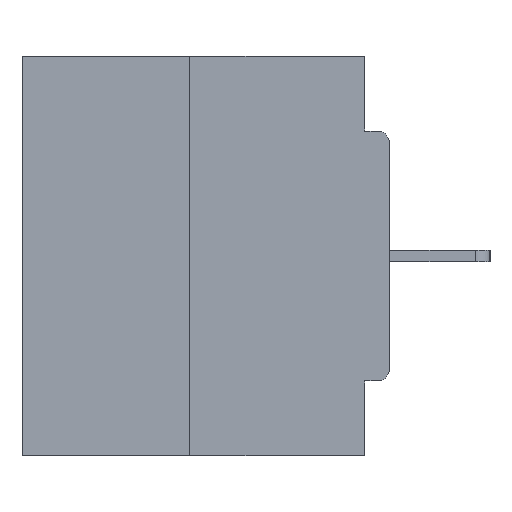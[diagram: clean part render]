
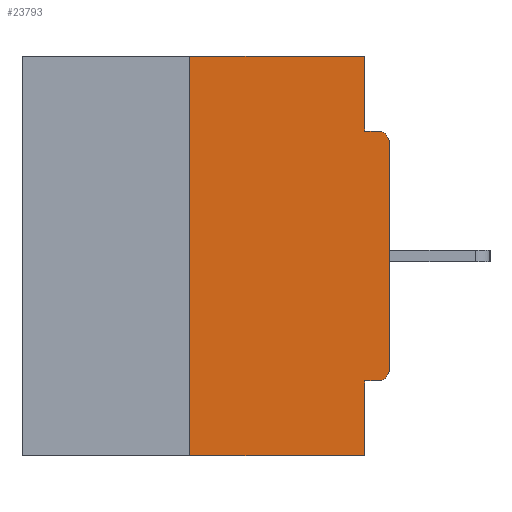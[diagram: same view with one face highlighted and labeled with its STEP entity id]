
A CAD part, left-side view. The second image highlights one B-rep face of the part: STEP entity #23793.
In plain terms, the highlighted planar face has unit normal (-1, 0, 0).
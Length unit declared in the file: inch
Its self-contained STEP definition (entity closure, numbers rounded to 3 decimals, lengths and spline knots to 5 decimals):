
#440 = EDGE_CURVE ( 'NONE', #18291, #3033, #17135, .T. ) ;
#484 = ORIENTED_EDGE ( 'NONE', *, *, #12071, .F. ) ;
#858 = VERTEX_POINT ( 'NONE', #8418 ) ;
#1251 = ORIENTED_EDGE ( 'NONE', *, *, #30407, .F. ) ;
#1846 = CARTESIAN_POINT ( 'NONE',  ( 0., 0.031, -0.5 ) ) ;
#2391 = CARTESIAN_POINT ( 'NONE',  ( 0., 0., -0.1085 ) ) ;
#3033 = VERTEX_POINT ( 'NONE', #1846 ) ;
#3339 = EDGE_CURVE ( 'NONE', #17771, #24456, #18511, .T. ) ;
#3683 = VECTOR ( 'NONE', #10704, 39.37008 ) ;
#3714 = CARTESIAN_POINT ( 'NONE',  ( 0., 0.015, -0.1085 ) ) ;
#4414 = ORIENTED_EDGE ( 'NONE', *, *, #12918, .T. ) ;
#4760 = CARTESIAN_POINT ( 'NONE',  ( 0., 0.46, 0. ) ) ;
#4828 = LINE ( 'NONE', #17891, #10597 ) ;
#4880 = CARTESIAN_POINT ( 'NONE',  ( 0., 0.25, 0. ) ) ;
#5171 = ORIENTED_EDGE ( 'NONE', *, *, #12303, .F. ) ;
#6205 = AXIS2_PLACEMENT_3D ( 'NONE', #26449, #26445, #26379 ) ;
#6224 = DIRECTION ( 'NONE',  ( 0., 0., -1. ) ) ;
#6331 = ORIENTED_EDGE ( 'NONE', *, *, #3339, .F. ) ;
#6459 = VECTOR ( 'NONE', #11971, 39.37008 ) ;
#7105 = ORIENTED_EDGE ( 'NONE', *, *, #440, .T. ) ;
#7230 = DIRECTION ( 'NONE',  ( 1., 0., 0. ) ) ;
#7357 = EDGE_CURVE ( 'NONE', #858, #25612, #29473, .T. ) ;
#7960 = EDGE_LOOP ( 'NONE', ( #6331, #484, #7105, #1251, #27977, #28705, #10176, #4414, #5171, #18187 ) ) ;
#8163 = VERTEX_POINT ( 'NONE', #8510 ) ;
#8179 = DIRECTION ( 'NONE',  ( 0., -1., 0. ) ) ;
#8418 = CARTESIAN_POINT ( 'NONE',  ( 0., 0.015, -0.4065 ) ) ;
#8510 = CARTESIAN_POINT ( 'NONE',  ( 0., 0.031, -0.4065 ) ) ;
#10176 = ORIENTED_EDGE ( 'NONE', *, *, #27878, .T. ) ;
#10597 = VECTOR ( 'NONE', #8179, 39.37008 ) ;
#10667 = VECTOR ( 'NONE', #26387, 39.37008 ) ;
#10704 = DIRECTION ( 'NONE',  ( 0., 1., 0. ) ) ;
#11031 = LINE ( 'NONE', #25330, #3683 ) ;
#11694 = EDGE_CURVE ( 'NONE', #858, #8163, #11031, .T. ) ;
#11783 = LINE ( 'NONE', #4880, #17455 ) ;
#11971 = DIRECTION ( 'NONE',  ( 0., 0., -1. ) ) ;
#12055 = VERTEX_POINT ( 'NONE', #14621 ) ;
#12056 = CARTESIAN_POINT ( 'NONE',  ( 0., 0.46, 0. ) ) ;
#12071 = EDGE_CURVE ( 'NONE', #18291, #17771, #11783, .T. ) ;
#12122 = DIRECTION ( 'NONE',  ( 0., 0., 1. ) ) ;
#12216 = CARTESIAN_POINT ( 'NONE',  ( 0., 0.031, 0. ) ) ;
#12303 = EDGE_CURVE ( 'NONE', #19927, #12055, #4828, .T. ) ;
#12918 = EDGE_CURVE ( 'NONE', #16972, #12055, #25348, .T. ) ;
#14215 = CARTESIAN_POINT ( 'NONE',  ( 0., 0.25, 0. ) ) ;
#14621 = CARTESIAN_POINT ( 'NONE',  ( 0., 0.015, -0.0935 ) ) ;
#15422 = DIRECTION ( 'NONE',  ( 0., -1., 0. ) ) ;
#16074 = CARTESIAN_POINT ( 'NONE',  ( 0., 0.25, -0.5 ) ) ;
#16972 = VERTEX_POINT ( 'NONE', #2391 ) ;
#17135 = LINE ( 'NONE', #25117, #10667 ) ;
#17455 = VECTOR ( 'NONE', #21977, 39.37008 ) ;
#17771 = VERTEX_POINT ( 'NONE', #14215 ) ;
#17891 = CARTESIAN_POINT ( 'NONE',  ( 0., 0., -0.0935 ) ) ;
#18096 = VECTOR ( 'NONE', #12122, 39.37008 ) ;
#18187 = ORIENTED_EDGE ( 'NONE', *, *, #19169, .F. ) ;
#18291 = VERTEX_POINT ( 'NONE', #16074 ) ;
#18511 = LINE ( 'NONE', #12056, #31262 ) ;
#18854 = LINE ( 'NONE', #31361, #18096 ) ;
#19169 = EDGE_CURVE ( 'NONE', #24456, #19927, #21988, .T. ) ;
#19278 = CARTESIAN_POINT ( 'NONE',  ( 0., 0.031, -0.5 ) ) ;
#19344 = FACE_OUTER_BOUND ( 'NONE', #7960, .T. ) ;
#19397 = PLANE ( 'NONE',  #20259 ) ;
#19447 = LINE ( 'NONE', #19278, #6459 ) ;
#19927 = VERTEX_POINT ( 'NONE', #20457 ) ;
#20259 = AXIS2_PLACEMENT_3D ( 'NONE', #4760, #7230, #24256 ) ;
#20457 = CARTESIAN_POINT ( 'NONE',  ( 0., 0.031, -0.0935 ) ) ;
#20851 = DIRECTION ( 'NONE',  ( -1., 0., 0. ) ) ;
#21977 = DIRECTION ( 'NONE',  ( 0., 0., 1. ) ) ;
#21988 = LINE ( 'NONE', #12216, #27566 ) ;
#22565 = CARTESIAN_POINT ( 'NONE',  ( 0., 0., -0.3915 ) ) ;
#23793 = ADVANCED_FACE ( 'NONE', ( #19344 ), #19397, .F. ) ;
#24256 = DIRECTION ( 'NONE',  ( 0., 0., -1. ) ) ;
#24456 = VERTEX_POINT ( 'NONE', #27337 ) ;
#25117 = CARTESIAN_POINT ( 'NONE',  ( 0., 0.46, -0.5 ) ) ;
#25330 = CARTESIAN_POINT ( 'NONE',  ( 0., 0., -0.4065 ) ) ;
#25348 = CIRCLE ( 'NONE', #31241, 0.015 ) ;
#25612 = VERTEX_POINT ( 'NONE', #22565 ) ;
#26379 = DIRECTION ( 'NONE',  ( 0., 0., -1. ) ) ;
#26387 = DIRECTION ( 'NONE',  ( 0., -1., 0. ) ) ;
#26445 = DIRECTION ( 'NONE',  ( -1., 0., 0. ) ) ;
#26449 = CARTESIAN_POINT ( 'NONE',  ( 0., 0.015, -0.3915 ) ) ;
#27337 = CARTESIAN_POINT ( 'NONE',  ( 0., 0.031, 0. ) ) ;
#27566 = VECTOR ( 'NONE', #31347, 39.37008 ) ;
#27878 = EDGE_CURVE ( 'NONE', #25612, #16972, #18854, .T. ) ;
#27977 = ORIENTED_EDGE ( 'NONE', *, *, #11694, .F. ) ;
#28705 = ORIENTED_EDGE ( 'NONE', *, *, #7357, .T. ) ;
#29473 = CIRCLE ( 'NONE', #6205, 0.015 ) ;
#30407 = EDGE_CURVE ( 'NONE', #8163, #3033, #19447, .T. ) ;
#31241 = AXIS2_PLACEMENT_3D ( 'NONE', #3714, #20851, #6224 ) ;
#31262 = VECTOR ( 'NONE', #15422, 39.37008 ) ;
#31347 = DIRECTION ( 'NONE',  ( 0., 0., -1. ) ) ;
#31361 = CARTESIAN_POINT ( 'NONE',  ( 0., 0., 0. ) ) ;
